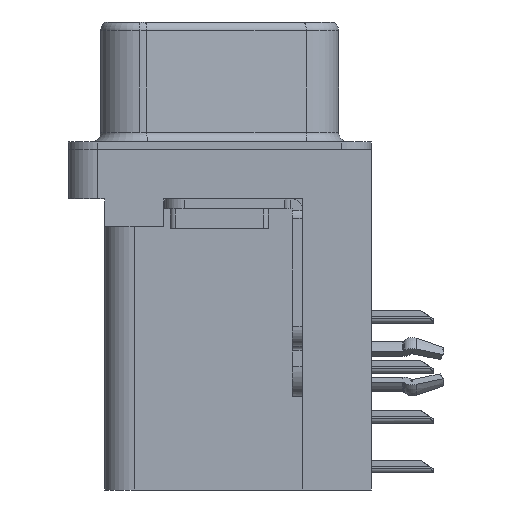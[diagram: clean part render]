
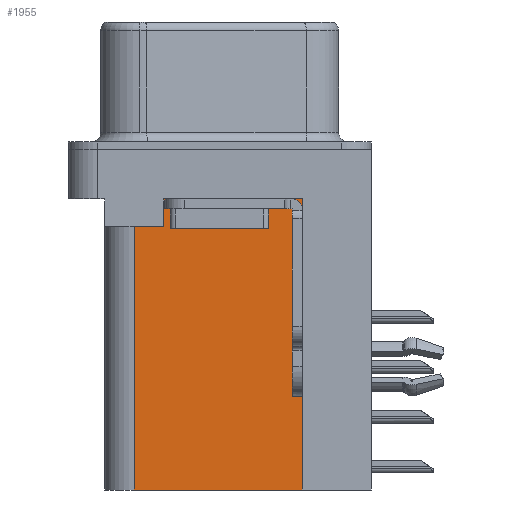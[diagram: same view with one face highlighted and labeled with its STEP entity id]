
A CAD part, left-side view. The second image highlights one B-rep face of the part: STEP entity #1955.
In plain terms, the highlighted planar face has unit normal (-1, 0, 0).
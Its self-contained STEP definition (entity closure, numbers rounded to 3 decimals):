
#53 = VERTEX_POINT ( 'NONE', #32015 ) ;
#1502 = FACE_OUTER_BOUND ( 'NONE', #33897, .T. ) ;
#1955 = ADVANCED_FACE ( 'NONE', ( #1502 ), #9519, .F. ) ;
#2274 = DIRECTION ( 'NONE',  ( 0., 0., 1. ) ) ;
#3668 = EDGE_CURVE ( 'NONE', #10958, #10075, #40457, .T. ) ;
#5444 = CARTESIAN_POINT ( 'NONE',  ( 3.75, -4.2, -17.3 ) ) ;
#7444 = DIRECTION ( 'NONE',  ( 0., 0., 1. ) ) ;
#9519 = PLANE ( 'NONE',  #40548 ) ;
#9725 = EDGE_CURVE ( 'NONE', #53, #22228, #32298, .T. ) ;
#10065 = ORIENTED_EDGE ( 'NONE', *, *, #25947, .F. ) ;
#10075 = VERTEX_POINT ( 'NONE', #28257 ) ;
#10958 = VERTEX_POINT ( 'NONE', #37781 ) ;
#11065 = ORIENTED_EDGE ( 'NONE', *, *, #25749, .F. ) ;
#12163 = ORIENTED_EDGE ( 'NONE', *, *, #9725, .T. ) ;
#13126 = CARTESIAN_POINT ( 'NONE',  ( 3.75, 4.35, -3.9 ) ) ;
#14312 = ORIENTED_EDGE ( 'NONE', *, *, #18164, .T. ) ;
#18164 = EDGE_CURVE ( 'NONE', #10075, #53, #18429, .T. ) ;
#18310 = VECTOR ( 'NONE', #34240, 1000. ) ;
#18429 = LINE ( 'NONE', #31059, #18310 ) ;
#22228 = VERTEX_POINT ( 'NONE', #13126 ) ;
#24259 = CARTESIAN_POINT ( 'NONE',  ( 3.75, -4.2, -17.3 ) ) ;
#25616 = VERTEX_POINT ( 'NONE', #5444 ) ;
#25749 = EDGE_CURVE ( 'NONE', #37106, #22228, #42303, .T. ) ;
#25947 = EDGE_CURVE ( 'NONE', #25616, #37106, #41164, .T. ) ;
#26007 = EDGE_CURVE ( 'NONE', #25616, #10958, #40551, .T. ) ;
#27005 = DIRECTION ( 'NONE',  ( 0., 1., 0. ) ) ;
#27015 = CARTESIAN_POINT ( 'NONE',  ( 3.75, -4.2, -2.5 ) ) ;
#27706 = CARTESIAN_POINT ( 'NONE',  ( 3.75, -4.2, -17.3 ) ) ;
#28257 = CARTESIAN_POINT ( 'NONE',  ( 3.75, 2.85, -2.5 ) ) ;
#29721 = CARTESIAN_POINT ( 'NONE',  ( 3.75, 4.35, -17.3 ) ) ;
#30848 = DIRECTION ( 'NONE',  ( 0., 1., 0. ) ) ;
#31059 = CARTESIAN_POINT ( 'NONE',  ( 3.75, 2.85, -3.9 ) ) ;
#32015 = CARTESIAN_POINT ( 'NONE',  ( 3.75, 2.85, -3.9 ) ) ;
#32126 = VECTOR ( 'NONE', #38572, 1000. ) ;
#32298 = LINE ( 'NONE', #35501, #32126 ) ;
#32608 = CARTESIAN_POINT ( 'NONE',  ( 3.75, -4.2, -17.3 ) ) ;
#32648 = DIRECTION ( 'NONE',  ( 1., 0., 0. ) ) ;
#32657 = DIRECTION ( 'NONE',  ( 0., 1., 0. ) ) ;
#33897 = EDGE_LOOP ( 'NONE', ( #36979, #14312, #12163, #11065, #10065, #39929 ) ) ;
#34240 = DIRECTION ( 'NONE',  ( 0., 0., -1. ) ) ;
#35501 = CARTESIAN_POINT ( 'NONE',  ( 3.75, 0., -3.9 ) ) ;
#36979 = ORIENTED_EDGE ( 'NONE', *, *, #3668, .T. ) ;
#37063 = CARTESIAN_POINT ( 'NONE',  ( 3.75, 4.35, -17.3 ) ) ;
#37106 = VERTEX_POINT ( 'NONE', #37063 ) ;
#37781 = CARTESIAN_POINT ( 'NONE',  ( 3.75, -4.2, -2.5 ) ) ;
#38572 = DIRECTION ( 'NONE',  ( 0., 1., 0. ) ) ;
#39929 = ORIENTED_EDGE ( 'NONE', *, *, #26007, .T. ) ;
#40344 = VECTOR ( 'NONE', #27005, 1000. ) ;
#40357 = VECTOR ( 'NONE', #7444, 1000. ) ;
#40457 = LINE ( 'NONE', #27015, #40344 ) ;
#40548 = AXIS2_PLACEMENT_3D ( 'NONE', #32608, #32648, #32657 ) ;
#40551 = LINE ( 'NONE', #27706, #40357 ) ;
#40599 = VECTOR ( 'NONE', #30848, 1000. ) ;
#41164 = LINE ( 'NONE', #24259, #40599 ) ;
#42303 = LINE ( 'NONE', #29721, #42506 ) ;
#42506 = VECTOR ( 'NONE', #2274, 1000. ) ;
